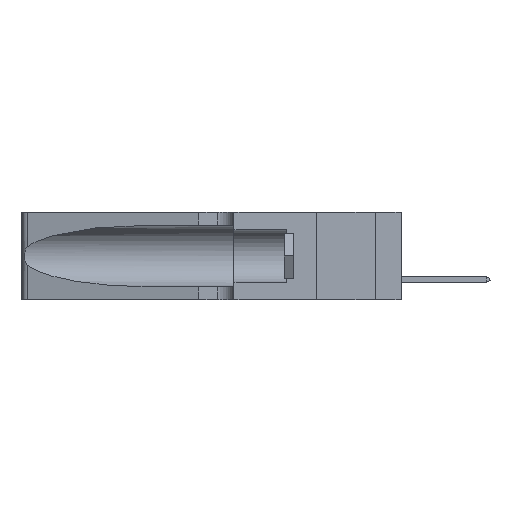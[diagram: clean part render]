
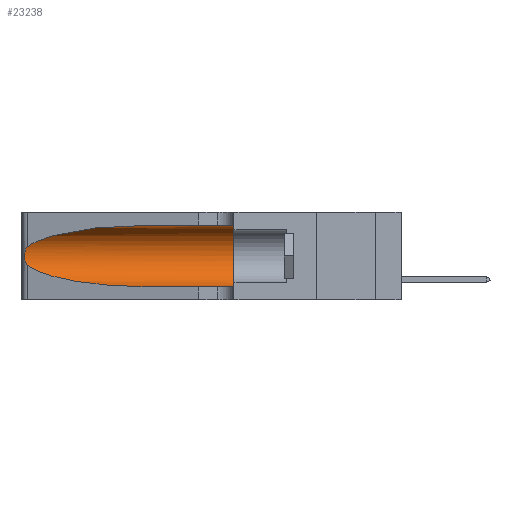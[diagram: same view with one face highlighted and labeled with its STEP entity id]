
A CAD part, left-side view. The second image highlights one B-rep face of the part: STEP entity #23238.
In plain terms, the highlighted cylindrical face has radius 3.308 mm (diameter 6.617 mm), a partial arc.
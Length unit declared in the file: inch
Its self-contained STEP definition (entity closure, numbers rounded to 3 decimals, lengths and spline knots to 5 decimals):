
#1518 = CARTESIAN_POINT ( 'NONE',  ( 0.25639, 1.23186, 0.15144 ) ) ;
#2967 = CARTESIAN_POINT ( 'NONE',  ( 0.18966, 0.96281, 0.31525 ) ) ;
#4175 = DIRECTION ( 'NONE',  ( 0., -1., 0. ) ) ;
#4503 = VERTEX_POINT ( 'NONE', #25148 ) ;
#4522 = CARTESIAN_POINT ( 'NONE',  ( 0.1305, 1.61858, 0.185 ) ) ;
#5956 = CARTESIAN_POINT ( 'NONE',  ( 0.1305, 0.35, 0.185 ) ) ;
#6942 = CARTESIAN_POINT ( 'NONE',  ( 0.2373, 1.15595, 0.28018 ) ) ;
#7302 = CARTESIAN_POINT ( 'NONE',  ( 0.25639, 1.23184, 0.21858 ) ) ;
#7613 = CARTESIAN_POINT ( 'NONE',  ( 0.25854, 1.2359, 0.20912 ) ) ;
#7758 = CARTESIAN_POINT ( 'NONE',  ( 0.26017, 1.23833, 0.17102 ) ) ;
#8357 = CYLINDRICAL_SURFACE ( 'NONE', #18327, 0.13025 ) ;
#8808 = ORIENTED_EDGE ( 'NONE', *, *, #27451, .F. ) ;
#8829 = VERTEX_POINT ( 'NONE', #44298 ) ;
#8830 = DIRECTION ( 'NONE',  ( 0., 0., -1. ) ) ;
#9939 = CARTESIAN_POINT ( 'NONE',  ( 0.1305, 1.61858, 0.05475 ) ) ;
#10031 = CARTESIAN_POINT ( 'NONE',  ( 0.25487, 1.22718, 0.14631 ) ) ;
#10578 = CARTESIAN_POINT ( 'NONE',  ( 0.25487, 1.22718, 0.22369 ) ) ;
#11003 =( BOUNDED_CURVE ( )  B_SPLINE_CURVE ( 3, ( #46156, #21083, #24393, #46630 ),
 .UNSPECIFIED., .F., .F. ) 
 B_SPLINE_CURVE_WITH_KNOTS ( ( 4, 4 ),
 ( 3.44316, 4.71239 ),
 .UNSPECIFIED. ) 
 CURVE ( )  GEOMETRIC_REPRESENTATION_ITEM ( )  RATIONAL_B_SPLINE_CURVE ( ( 1., 0.87, 0.87, 1. ) ) 
 REPRESENTATION_ITEM ( '' )  );
#11412 = EDGE_CURVE ( 'NONE', #8829, #11719, #16497, .T. ) ;
#11662 = CARTESIAN_POINT ( 'NONE',  ( 0.26018, 1.23835, 0.19895 ) ) ;
#11719 = VERTEX_POINT ( 'NONE', #10031 ) ;
#12176 = EDGE_CURVE ( 'NONE', #32871, #13069, #16304, .T. ) ;
#12450 = CARTESIAN_POINT ( 'NONE',  ( 0.25555, 1.22993, 0.14849 ) ) ;
#12860 = CARTESIAN_POINT ( 'NONE',  ( 0.1305, 0.35, 0.05475 ) ) ;
#13069 = VERTEX_POINT ( 'NONE', #12860 ) ;
#13397 = DIRECTION ( 'NONE',  ( 0., 0., 1. ) ) ;
#14572 = FACE_OUTER_BOUND ( 'NONE', #28044, .T. ) ;
#15421 = CARTESIAN_POINT ( 'NONE',  ( 0.26075, 1.23896, 0.178 ) ) ;
#15907 = DIRECTION ( 'NONE',  ( 0., -1., 0. ) ) ;
#16304 = CIRCLE ( 'NONE', #30761, 0.13025 ) ;
#16497 = B_SPLINE_CURVE_WITH_KNOTS ( 'NONE', 3,
 ( #34188, #28172, #7302, #21926, #7613, #11662, #22528, #15421, #7758, #32979, #43933, #1518, #12450, #30634 ),
 .UNSPECIFIED., .F., .F.,
 ( 4, 2, 2, 2, 2, 2, 4 ),
 ( 0., 0.00027, 0.00053, 0.00107, 0.0016, 0.00187, 0.00214 ),
 .UNSPECIFIED. ) ;
#16979 = VECTOR ( 'NONE', #4175, 39.37008 ) ;
#18327 = AXIS2_PLACEMENT_3D ( 'NONE', #4522, #15907, #8830 ) ;
#20737 = ORIENTED_EDGE ( 'NONE', *, *, #11412, .T. ) ;
#21083 = CARTESIAN_POINT ( 'NONE',  ( 0.2373, 1.15595, 0.08982 ) ) ;
#21399 = VERTEX_POINT ( 'NONE', #22857 ) ;
#21926 = CARTESIAN_POINT ( 'NONE',  ( 0.25787, 1.23484, 0.2124 ) ) ;
#22132 = EDGE_CURVE ( 'NONE', #21399, #13069, #25394, .T. ) ;
#22528 = CARTESIAN_POINT ( 'NONE',  ( 0.26075, 1.23896, 0.19203 ) ) ;
#22857 = CARTESIAN_POINT ( 'NONE',  ( 0.1305, 0.72297, 0.05475 ) ) ;
#23238 = ADVANCED_FACE ( 'NONE', ( #14572 ), #8357, .F. ) ;
#24393 = CARTESIAN_POINT ( 'NONE',  ( 0.18966, 0.96281, 0.05475 ) ) ;
#24760 = CARTESIAN_POINT ( 'NONE',  ( 0.1305, 0.35, 0.31525 ) ) ;
#24832 = ORIENTED_EDGE ( 'NONE', *, *, #42152, .T. ) ;
#25148 = CARTESIAN_POINT ( 'NONE',  ( 0.1305, 0.72297, 0.31525 ) ) ;
#25394 = LINE ( 'NONE', #9939, #43534 ) ;
#27451 = EDGE_CURVE ( 'NONE', #4503, #32871, #39665, .T. ) ;
#28044 = EDGE_LOOP ( 'NONE', ( #24832, #20737, #36081, #33447, #30559, #8808 ) ) ;
#28172 = CARTESIAN_POINT ( 'NONE',  ( 0.25555, 1.22994, 0.2215 ) ) ;
#28589 = CARTESIAN_POINT ( 'NONE',  ( 0.1305, 0.72297, 0.31525 ) ) ;
#30559 = ORIENTED_EDGE ( 'NONE', *, *, #12176, .F. ) ;
#30634 = CARTESIAN_POINT ( 'NONE',  ( 0.25487, 1.22718, 0.14631 ) ) ;
#30761 = AXIS2_PLACEMENT_3D ( 'NONE', #5956, #34875, #13397 ) ;
#32871 = VERTEX_POINT ( 'NONE', #24760 ) ;
#32979 = CARTESIAN_POINT ( 'NONE',  ( 0.25856, 1.23593, 0.16098 ) ) ;
#33447 = ORIENTED_EDGE ( 'NONE', *, *, #22132, .T. ) ;
#34188 = CARTESIAN_POINT ( 'NONE',  ( 0.25487, 1.22718, 0.22369 ) ) ;
#34875 = DIRECTION ( 'NONE',  ( 0., 1., 0. ) ) ;
#36081 = ORIENTED_EDGE ( 'NONE', *, *, #44887, .T. ) ;
#36901 = CARTESIAN_POINT ( 'NONE',  ( 0.1305, 1.61858, 0.31525 ) ) ;
#38649 = DIRECTION ( 'NONE',  ( 0., -1., 0. ) ) ;
#39467 =( BOUNDED_CURVE ( )  B_SPLINE_CURVE ( 3, ( #28589, #2967, #6942, #10578 ),
 .UNSPECIFIED., .F., .F. ) 
 B_SPLINE_CURVE_WITH_KNOTS ( ( 4, 4 ),
 ( 1.5708, 2.84003 ),
 .UNSPECIFIED. ) 
 CURVE ( )  GEOMETRIC_REPRESENTATION_ITEM ( )  RATIONAL_B_SPLINE_CURVE ( ( 1., 0.87, 0.87, 1. ) ) 
 REPRESENTATION_ITEM ( '' )  );
#39665 = LINE ( 'NONE', #36901, #16979 ) ;
#42152 = EDGE_CURVE ( 'NONE', #4503, #8829, #39467, .T. ) ;
#43534 = VECTOR ( 'NONE', #38649, 39.37008 ) ;
#43933 = CARTESIAN_POINT ( 'NONE',  ( 0.25789, 1.23486, 0.15765 ) ) ;
#44298 = CARTESIAN_POINT ( 'NONE',  ( 0.25487, 1.22718, 0.22369 ) ) ;
#44887 = EDGE_CURVE ( 'NONE', #11719, #21399, #11003, .T. ) ;
#46156 = CARTESIAN_POINT ( 'NONE',  ( 0.25487, 1.22718, 0.14631 ) ) ;
#46630 = CARTESIAN_POINT ( 'NONE',  ( 0.1305, 0.72297, 0.05475 ) ) ;
